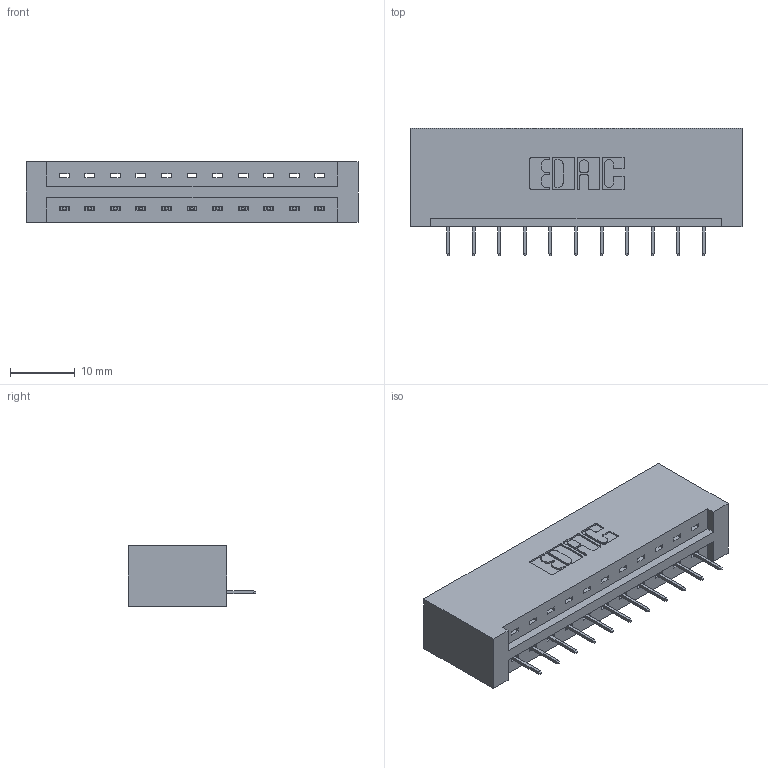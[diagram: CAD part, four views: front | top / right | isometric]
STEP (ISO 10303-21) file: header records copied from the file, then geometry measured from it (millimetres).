
FILE_DESCRIPTION (( 'STEP AP203' ), '1' );
FILE_NAME ('337-011-524-101.STEP', '2018-08-04T01:19:37', ( '' ), ( '' ), 'SwSTEP 2.0', 'SolidWorks 2016', '' );
FILE_SCHEMA (( 'CONFIG_CONTROL_DESIGN' ));
Length unit declared in the file: inch
Products named in the file (3): 345-292-001_345-293-124; 337-011-524-101; 337 Part_No Mounting Lugs
Assembly tree (12 placements, depth 2):
  337-011-524-101
    337 Part_No Mounting Lugs
    345-292-001_345-293-124  x11
Bounding box: 51.46 x 19.69 x 9.4 mm (x, y, z)
Volume: 5655.8 mm3; surface area: 5501 mm2
Topology: 12 solids, 12 shells, 832 faces, 2399 edges, 1554 vertices
Faces by surface type: plane 638, cylinder 194
Entity records: 11983 total; most frequent: CARTESIAN_POINT 2091, ORIENTED_EDGE 2038, DIRECTION 1817, EDGE_CURVE 1019, LINE 903, VECTOR 903, VERTEX_POINT 674, AXIS2_PLACEMENT_3D 457
